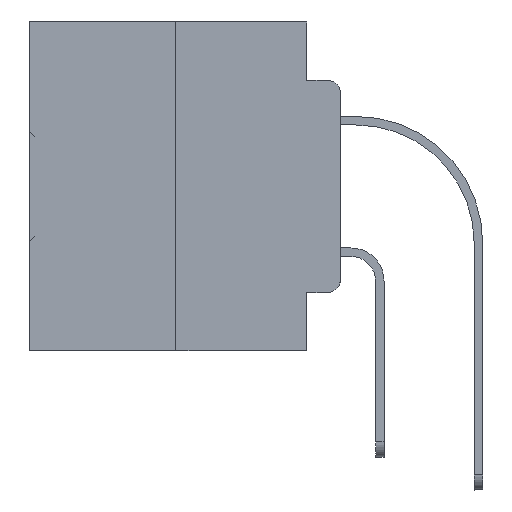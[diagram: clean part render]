
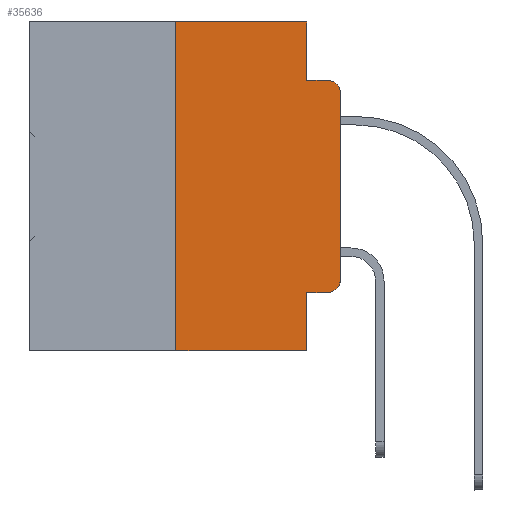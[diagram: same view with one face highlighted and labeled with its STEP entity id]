
A CAD part, left-side view. The second image highlights one B-rep face of the part: STEP entity #35636.
In plain terms, the highlighted planar face has unit normal (-1, 0, 0).
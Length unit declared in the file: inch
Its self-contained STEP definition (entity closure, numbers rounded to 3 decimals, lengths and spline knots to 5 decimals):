
#89 = CARTESIAN_POINT ( 'NONE',  ( 0., 0.473, -0.5 ) ) ;
#149 = EDGE_CURVE ( 'NONE', #22133, #32158, #3291, .T. ) ;
#969 = DIRECTION ( 'NONE',  ( 0., 0., -1. ) ) ;
#1084 = ORIENTED_EDGE ( 'NONE', *, *, #5417, .T. ) ;
#1099 = EDGE_CURVE ( 'NONE', #1679, #8121, #29360, .T. ) ;
#1226 = EDGE_CURVE ( 'NONE', #13568, #2871, #18978, .T. ) ;
#1248 = VERTEX_POINT ( 'NONE', #30272 ) ;
#1679 = VERTEX_POINT ( 'NONE', #35387 ) ;
#1776 = DIRECTION ( 'NONE',  ( 0., -1., 0. ) ) ;
#1862 = DIRECTION ( 'NONE',  ( 0., -1., 0. ) ) ;
#2164 = CIRCLE ( 'NONE', #9232, 0.02 ) ;
#2522 = CARTESIAN_POINT ( 'NONE',  ( 0., 0.051, 0. ) ) ;
#2582 = PLANE ( 'NONE',  #7620 ) ;
#2693 = CARTESIAN_POINT ( 'NONE',  ( 0., 0.473, 0. ) ) ;
#2871 = VERTEX_POINT ( 'NONE', #14775 ) ;
#3000 = CARTESIAN_POINT ( 'NONE',  ( 0., 0.02, -0.1085 ) ) ;
#3291 = CIRCLE ( 'NONE', #15710, 0.02 ) ;
#3570 = CARTESIAN_POINT ( 'NONE',  ( 0., 0.02, -0.4115 ) ) ;
#4726 = VECTOR ( 'NONE', #1862, 39.37008 ) ;
#4754 = EDGE_CURVE ( 'NONE', #1679, #13592, #25417, .T. ) ;
#5417 = EDGE_CURVE ( 'NONE', #20973, #22133, #21284, .T. ) ;
#5498 = EDGE_CURVE ( 'NONE', #32158, #1248, #9651, .T. ) ;
#6201 = ORIENTED_EDGE ( 'NONE', *, *, #35970, .F. ) ;
#6483 = CARTESIAN_POINT ( 'NONE',  ( 0., 0.051, 0. ) ) ;
#7071 = VECTOR ( 'NONE', #35810, 39.37008 ) ;
#7221 = CARTESIAN_POINT ( 'NONE',  ( 0., 0.051, -0.4115 ) ) ;
#7620 = AXIS2_PLACEMENT_3D ( 'NONE', #11456, #28649, #17186 ) ;
#8121 = VERTEX_POINT ( 'NONE', #19463 ) ;
#8419 = DIRECTION ( 'NONE',  ( 0., 0., -1. ) ) ;
#8672 = ORIENTED_EDGE ( 'NONE', *, *, #4754, .T. ) ;
#8774 = VECTOR ( 'NONE', #29560, 39.37008 ) ;
#9232 = AXIS2_PLACEMENT_3D ( 'NONE', #3000, #9276, #969 ) ;
#9276 = DIRECTION ( 'NONE',  ( -1., 0., 0. ) ) ;
#9457 = ORIENTED_EDGE ( 'NONE', *, *, #28911, .F. ) ;
#9651 = LINE ( 'NONE', #35166, #11849 ) ;
#9670 = CARTESIAN_POINT ( 'NONE',  ( 0., 0.051, -0.4115 ) ) ;
#9826 = DIRECTION ( 'NONE',  ( 0., 0., 1. ) ) ;
#10628 = LINE ( 'NONE', #2693, #28655 ) ;
#11073 = FACE_OUTER_BOUND ( 'NONE', #28245, .T. ) ;
#11182 = ORIENTED_EDGE ( 'NONE', *, *, #149, .T. ) ;
#11456 = CARTESIAN_POINT ( 'NONE',  ( 0., 0.473, 0. ) ) ;
#11688 = CARTESIAN_POINT ( 'NONE',  ( 0., 0.051, -0.5 ) ) ;
#11849 = VECTOR ( 'NONE', #9826, 39.37008 ) ;
#13513 = VERTEX_POINT ( 'NONE', #6483 ) ;
#13568 = VERTEX_POINT ( 'NONE', #31499 ) ;
#13592 = VERTEX_POINT ( 'NONE', #11688 ) ;
#14586 = DIRECTION ( 'NONE',  ( 0., 0., 1. ) ) ;
#14775 = CARTESIAN_POINT ( 'NONE',  ( 0., 0.02, -0.0885 ) ) ;
#15710 = AXIS2_PLACEMENT_3D ( 'NONE', #16776, #25249, #8419 ) ;
#15842 = CARTESIAN_POINT ( 'NONE',  ( 0., 0.051, -0.0885 ) ) ;
#16414 = ORIENTED_EDGE ( 'NONE', *, *, #30794, .T. ) ;
#16776 = CARTESIAN_POINT ( 'NONE',  ( 0., 0.02, -0.3915 ) ) ;
#17186 = DIRECTION ( 'NONE',  ( 0., 0., -1. ) ) ;
#18978 = LINE ( 'NONE', #15842, #32001 ) ;
#19164 = DIRECTION ( 'NONE',  ( 0., -1., 0. ) ) ;
#19463 = CARTESIAN_POINT ( 'NONE',  ( 0., 0.25, 0. ) ) ;
#20235 = ORIENTED_EDGE ( 'NONE', *, *, #5498, .T. ) ;
#20973 = VERTEX_POINT ( 'NONE', #9670 ) ;
#21284 = LINE ( 'NONE', #7221, #4726 ) ;
#21774 = LINE ( 'NONE', #27141, #8774 ) ;
#22133 = VERTEX_POINT ( 'NONE', #3570 ) ;
#22553 = ORIENTED_EDGE ( 'NONE', *, *, #1099, .F. ) ;
#23072 = CARTESIAN_POINT ( 'NONE',  ( 0., 0.25, 0. ) ) ;
#23556 = DIRECTION ( 'NONE',  ( 0., -1., 0. ) ) ;
#24233 = VECTOR ( 'NONE', #14586, 39.37008 ) ;
#25249 = DIRECTION ( 'NONE',  ( -1., 0., 0. ) ) ;
#25417 = LINE ( 'NONE', #89, #31517 ) ;
#27141 = CARTESIAN_POINT ( 'NONE',  ( 0., 0.051, 0. ) ) ;
#27310 = LINE ( 'NONE', #2522, #7071 ) ;
#28239 = EDGE_CURVE ( 'NONE', #13513, #13568, #21774, .T. ) ;
#28245 = EDGE_LOOP ( 'NONE', ( #20235, #16414, #36320, #33914, #9457, #22553, #8672, #6201, #1084, #11182 ) ) ;
#28649 = DIRECTION ( 'NONE',  ( 1., 0., 0. ) ) ;
#28655 = VECTOR ( 'NONE', #19164, 39.37008 ) ;
#28911 = EDGE_CURVE ( 'NONE', #8121, #13513, #10628, .T. ) ;
#29360 = LINE ( 'NONE', #23072, #24233 ) ;
#29560 = DIRECTION ( 'NONE',  ( 0., 0., -1. ) ) ;
#30042 = CARTESIAN_POINT ( 'NONE',  ( 0., 0., -0.3915 ) ) ;
#30272 = CARTESIAN_POINT ( 'NONE',  ( 0., 0., -0.1085 ) ) ;
#30794 = EDGE_CURVE ( 'NONE', #1248, #2871, #2164, .T. ) ;
#31499 = CARTESIAN_POINT ( 'NONE',  ( 0., 0.051, -0.0885 ) ) ;
#31517 = VECTOR ( 'NONE', #23556, 39.37008 ) ;
#32001 = VECTOR ( 'NONE', #1776, 39.37008 ) ;
#32158 = VERTEX_POINT ( 'NONE', #30042 ) ;
#33914 = ORIENTED_EDGE ( 'NONE', *, *, #28239, .F. ) ;
#35166 = CARTESIAN_POINT ( 'NONE',  ( 0., 0., 0. ) ) ;
#35387 = CARTESIAN_POINT ( 'NONE',  ( 0., 0.25, -0.5 ) ) ;
#35636 = ADVANCED_FACE ( 'NONE', ( #11073 ), #2582, .F. ) ;
#35810 = DIRECTION ( 'NONE',  ( 0., 0., -1. ) ) ;
#35970 = EDGE_CURVE ( 'NONE', #20973, #13592, #27310, .T. ) ;
#36320 = ORIENTED_EDGE ( 'NONE', *, *, #1226, .F. ) ;
